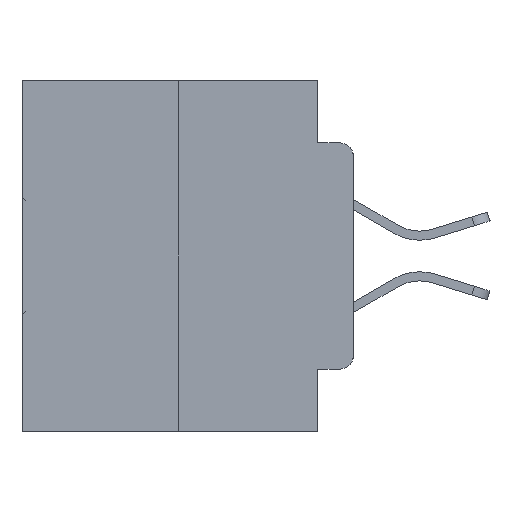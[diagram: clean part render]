
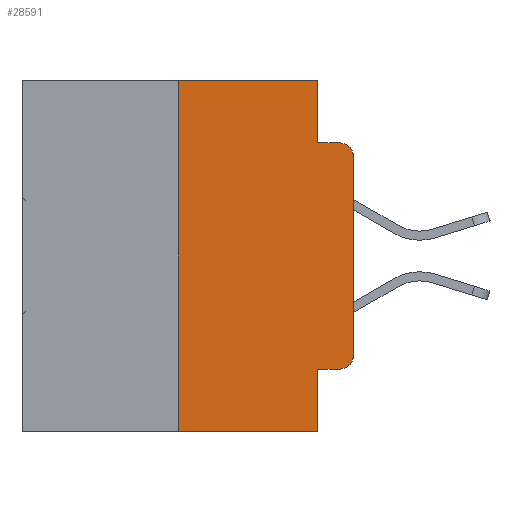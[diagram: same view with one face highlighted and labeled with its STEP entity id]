
A CAD part, left-side view. The second image highlights one B-rep face of the part: STEP entity #28591.
In plain terms, the highlighted planar face has unit normal (-1, 0, 0).
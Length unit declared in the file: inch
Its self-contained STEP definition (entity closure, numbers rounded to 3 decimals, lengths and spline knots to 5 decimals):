
#535 = VERTEX_POINT ( 'NONE', #4857 ) ;
#610 = LINE ( 'NONE', #27445, #30501 ) ;
#759 = VERTEX_POINT ( 'NONE', #19640 ) ;
#979 = CARTESIAN_POINT ( 'NONE',  ( 0., 0.051, 0. ) ) ;
#1594 = EDGE_CURVE ( 'NONE', #6956, #535, #27935, .T. ) ;
#1928 = CARTESIAN_POINT ( 'NONE',  ( 0., 0.051, 0. ) ) ;
#2286 = CARTESIAN_POINT ( 'NONE',  ( 0., 0.25, -0.5 ) ) ;
#3864 = LINE ( 'NONE', #19963, #28770 ) ;
#3867 = PLANE ( 'NONE',  #6615 ) ;
#4465 = DIRECTION ( 'NONE',  ( 0., 0., -1. ) ) ;
#4628 = ORIENTED_EDGE ( 'NONE', *, *, #12163, .T. ) ;
#4659 = ORIENTED_EDGE ( 'NONE', *, *, #13795, .T. ) ;
#4844 = VECTOR ( 'NONE', #20420, 39.37008 ) ;
#4857 = CARTESIAN_POINT ( 'NONE',  ( 0., 0., -0.3915 ) ) ;
#4969 = ORIENTED_EDGE ( 'NONE', *, *, #15365, .F. ) ;
#4981 = CARTESIAN_POINT ( 'NONE',  ( 0., 0.02, -0.4115 ) ) ;
#5126 = ORIENTED_EDGE ( 'NONE', *, *, #21783, .F. ) ;
#5499 = ORIENTED_EDGE ( 'NONE', *, *, #16788, .F. ) ;
#5633 = ORIENTED_EDGE ( 'NONE', *, *, #23387, .F. ) ;
#6232 = CARTESIAN_POINT ( 'NONE',  ( 0., 0.051, -0.4115 ) ) ;
#6515 = CARTESIAN_POINT ( 'NONE',  ( 0., 0.473, 0. ) ) ;
#6615 = AXIS2_PLACEMENT_3D ( 'NONE', #6515, #23367, #9011 ) ;
#6852 = ORIENTED_EDGE ( 'NONE', *, *, #8072, .T. ) ;
#6928 = VECTOR ( 'NONE', #21216, 39.37008 ) ;
#6956 = VERTEX_POINT ( 'NONE', #4981 ) ;
#6969 = ORIENTED_EDGE ( 'NONE', *, *, #29739, .F. ) ;
#7611 = ORIENTED_EDGE ( 'NONE', *, *, #31291, .T. ) ;
#7802 = EDGE_LOOP ( 'NONE', ( #4628, #4659, #4969, #5126, #5499, #5633, #6852, #6969, #7611, #8006 ) ) ;
#7856 = DIRECTION ( 'NONE',  ( 0., -1., 0. ) ) ;
#8006 = ORIENTED_EDGE ( 'NONE', *, *, #1594, .T. ) ;
#8072 = EDGE_CURVE ( 'NONE', #25241, #9045, #26076, .T. ) ;
#8150 = VECTOR ( 'NONE', #4465, 39.37008 ) ;
#9011 = DIRECTION ( 'NONE',  ( 0., 0., -1. ) ) ;
#9038 = VERTEX_POINT ( 'NONE', #28552 ) ;
#9045 = VERTEX_POINT ( 'NONE', #30902 ) ;
#9186 = VERTEX_POINT ( 'NONE', #14880 ) ;
#11687 = CARTESIAN_POINT ( 'NONE',  ( 0., 0.473, -0.5 ) ) ;
#12066 = CARTESIAN_POINT ( 'NONE',  ( 0., 0.02, -0.1085 ) ) ;
#12163 = EDGE_CURVE ( 'NONE', #535, #9038, #25234, .T. ) ;
#12305 = VERTEX_POINT ( 'NONE', #27886 ) ;
#12467 = CIRCLE ( 'NONE', #19299, 0.02 ) ;
#13354 = LINE ( 'NONE', #6232, #18194 ) ;
#13595 = DIRECTION ( 'NONE',  ( 0., -1., 0. ) ) ;
#13633 = CARTESIAN_POINT ( 'NONE',  ( 0., 0.02, -0.0885 ) ) ;
#13795 = EDGE_CURVE ( 'NONE', #9038, #30749, #12467, .T. ) ;
#14489 = DIRECTION ( 'NONE',  ( 0., 0., -1. ) ) ;
#14880 = CARTESIAN_POINT ( 'NONE',  ( 0., 0.25, 0. ) ) ;
#15365 = EDGE_CURVE ( 'NONE', #20692, #30749, #3864, .T. ) ;
#16788 = EDGE_CURVE ( 'NONE', #9186, #12305, #610, .T. ) ;
#16996 = LINE ( 'NONE', #979, #4844 ) ;
#18194 = VECTOR ( 'NONE', #13595, 39.37008 ) ;
#18886 = VECTOR ( 'NONE', #24595, 39.37008 ) ;
#19299 = AXIS2_PLACEMENT_3D ( 'NONE', #12066, #28757, #14489 ) ;
#19640 = CARTESIAN_POINT ( 'NONE',  ( 0., 0.051, -0.4115 ) ) ;
#19963 = CARTESIAN_POINT ( 'NONE',  ( 0., 0.051, -0.0885 ) ) ;
#20420 = DIRECTION ( 'NONE',  ( 0., 0., -1. ) ) ;
#20692 = VERTEX_POINT ( 'NONE', #25997 ) ;
#21216 = DIRECTION ( 'NONE',  ( 0., -1., 0. ) ) ;
#21569 = VECTOR ( 'NONE', #23954, 39.37008 ) ;
#21637 = DIRECTION ( 'NONE',  ( 0., 0., -1. ) ) ;
#21783 = EDGE_CURVE ( 'NONE', #12305, #20692, #16996, .T. ) ;
#22151 = DIRECTION ( 'NONE',  ( -1., 0., 0. ) ) ;
#22187 = CARTESIAN_POINT ( 'NONE',  ( 0., 0.02, -0.3915 ) ) ;
#23367 = DIRECTION ( 'NONE',  ( 1., 0., 0. ) ) ;
#23387 = EDGE_CURVE ( 'NONE', #25241, #9186, #27872, .T. ) ;
#23954 = DIRECTION ( 'NONE',  ( 0., 0., 1. ) ) ;
#24595 = DIRECTION ( 'NONE',  ( 0., 0., 1. ) ) ;
#24638 = FACE_OUTER_BOUND ( 'NONE', #7802, .T. ) ;
#25234 = LINE ( 'NONE', #26849, #18886 ) ;
#25241 = VERTEX_POINT ( 'NONE', #2286 ) ;
#25772 = LINE ( 'NONE', #1928, #8150 ) ;
#25997 = CARTESIAN_POINT ( 'NONE',  ( 0., 0.051, -0.0885 ) ) ;
#26076 = LINE ( 'NONE', #11687, #6928 ) ;
#26849 = CARTESIAN_POINT ( 'NONE',  ( 0., 0., 0. ) ) ;
#27445 = CARTESIAN_POINT ( 'NONE',  ( 0., 0.473, 0. ) ) ;
#27872 = LINE ( 'NONE', #30959, #21569 ) ;
#27886 = CARTESIAN_POINT ( 'NONE',  ( 0., 0.051, 0. ) ) ;
#27935 = CIRCLE ( 'NONE', #28225, 0.02 ) ;
#28225 = AXIS2_PLACEMENT_3D ( 'NONE', #22187, #22151, #21637 ) ;
#28552 = CARTESIAN_POINT ( 'NONE',  ( 0., 0., -0.1085 ) ) ;
#28591 = ADVANCED_FACE ( 'NONE', ( #24638 ), #3867, .F. ) ;
#28757 = DIRECTION ( 'NONE',  ( -1., 0., 0. ) ) ;
#28770 = VECTOR ( 'NONE', #7856, 39.37008 ) ;
#29739 = EDGE_CURVE ( 'NONE', #759, #9045, #25772, .T. ) ;
#29844 = DIRECTION ( 'NONE',  ( 0., -1., 0. ) ) ;
#30501 = VECTOR ( 'NONE', #29844, 39.37008 ) ;
#30749 = VERTEX_POINT ( 'NONE', #13633 ) ;
#30902 = CARTESIAN_POINT ( 'NONE',  ( 0., 0.051, -0.5 ) ) ;
#30959 = CARTESIAN_POINT ( 'NONE',  ( 0., 0.25, 0. ) ) ;
#31291 = EDGE_CURVE ( 'NONE', #759, #6956, #13354, .T. ) ;
